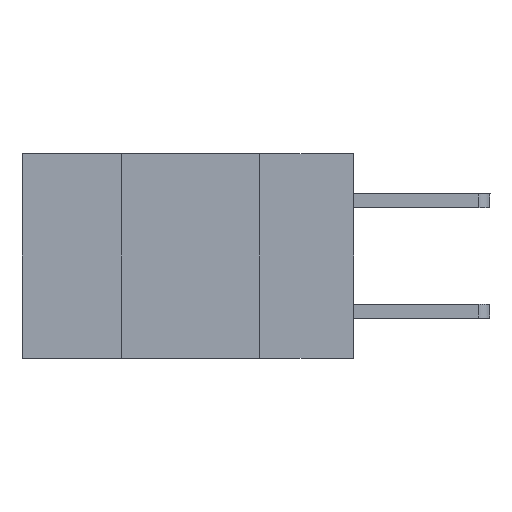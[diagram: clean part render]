
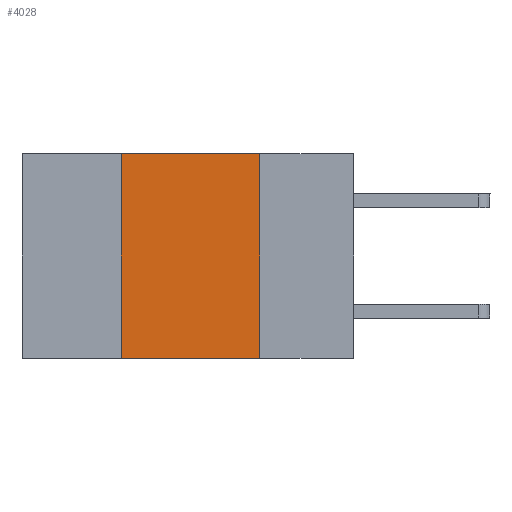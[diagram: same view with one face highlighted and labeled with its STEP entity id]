
A CAD part, left-side view. The second image highlights one B-rep face of the part: STEP entity #4028.
In plain terms, the highlighted planar face has unit normal (-1, 0, 0).
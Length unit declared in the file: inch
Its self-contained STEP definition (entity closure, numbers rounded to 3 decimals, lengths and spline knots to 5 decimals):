
#101 = VERTEX_POINT ( 'NONE', #8475 ) ;
#350 = CARTESIAN_POINT ( 'NONE',  ( 0., 0.6, -0.37 ) ) ;
#398 = DIRECTION ( 'NONE',  ( 0., -1., 0. ) ) ;
#546 = ORIENTED_EDGE ( 'NONE', *, *, #10736, .F. ) ;
#627 = ORIENTED_EDGE ( 'NONE', *, *, #13508, .F. ) ;
#759 = ORIENTED_EDGE ( 'NONE', *, *, #12233, .F. ) ;
#868 = ORIENTED_EDGE ( 'NONE', *, *, #12667, .T. ) ;
#1391 = DIRECTION ( 'NONE',  ( 0., -1., 0. ) ) ;
#1977 = CARTESIAN_POINT ( 'NONE',  ( 0., 0.42, 0. ) ) ;
#2005 = VERTEX_POINT ( 'NONE', #11139 ) ;
#2145 = PLANE ( 'NONE',  #14606 ) ;
#3218 = VERTEX_POINT ( 'NONE', #14215 ) ;
#3338 = DIRECTION ( 'NONE',  ( 1., 0., 0. ) ) ;
#4028 = ADVANCED_FACE ( 'NONE', ( #12853 ), #2145, .F. ) ;
#4878 = VECTOR ( 'NONE', #6192, 39.37008 ) ;
#5234 = LINE ( 'NONE', #9540, #4878 ) ;
#6192 = DIRECTION ( 'NONE',  ( 0., 0., -1. ) ) ;
#8260 = CARTESIAN_POINT ( 'NONE',  ( 0., 0.42, 0. ) ) ;
#8475 = CARTESIAN_POINT ( 'NONE',  ( 0., 0.17, 0. ) ) ;
#8642 = EDGE_LOOP ( 'NONE', ( #546, #627, #759, #868 ) ) ;
#8864 = VECTOR ( 'NONE', #1391, 39.37008 ) ;
#8890 = VECTOR ( 'NONE', #398, 39.37008 ) ;
#9247 = LINE ( 'NONE', #1977, #12229 ) ;
#9406 = CARTESIAN_POINT ( 'NONE',  ( 0., 0.6, 0. ) ) ;
#9540 = CARTESIAN_POINT ( 'NONE',  ( 0., 0.17, 0. ) ) ;
#10169 = CARTESIAN_POINT ( 'NONE',  ( 0., 0.6, 0. ) ) ;
#10736 = EDGE_CURVE ( 'NONE', #101, #2005, #5234, .T. ) ;
#11139 = CARTESIAN_POINT ( 'NONE',  ( 0., 0.17, -0.37 ) ) ;
#11282 = DIRECTION ( 'NONE',  ( 0., 0., -1. ) ) ;
#11302 = VERTEX_POINT ( 'NONE', #8260 ) ;
#11860 = LINE ( 'NONE', #350, #8890 ) ;
#12188 = LINE ( 'NONE', #9406, #8864 ) ;
#12229 = VECTOR ( 'NONE', #14372, 39.37008 ) ;
#12233 = EDGE_CURVE ( 'NONE', #3218, #11302, #9247, .T. ) ;
#12667 = EDGE_CURVE ( 'NONE', #3218, #2005, #11860, .T. ) ;
#12853 = FACE_OUTER_BOUND ( 'NONE', #8642, .T. ) ;
#13508 = EDGE_CURVE ( 'NONE', #11302, #101, #12188, .T. ) ;
#14215 = CARTESIAN_POINT ( 'NONE',  ( 0., 0.42, -0.37 ) ) ;
#14372 = DIRECTION ( 'NONE',  ( 0., 0., 1. ) ) ;
#14606 = AXIS2_PLACEMENT_3D ( 'NONE', #10169, #3338, #11282 ) ;
